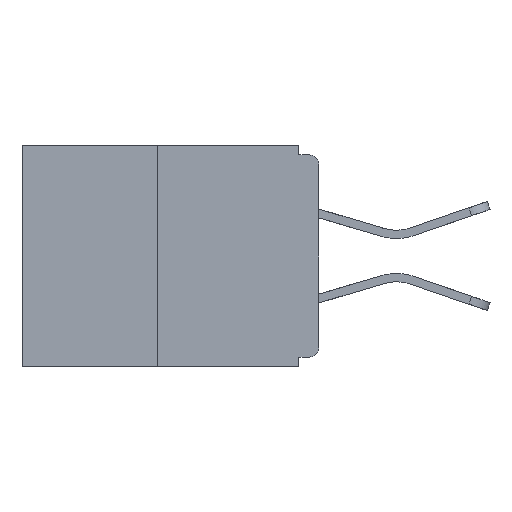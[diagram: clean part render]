
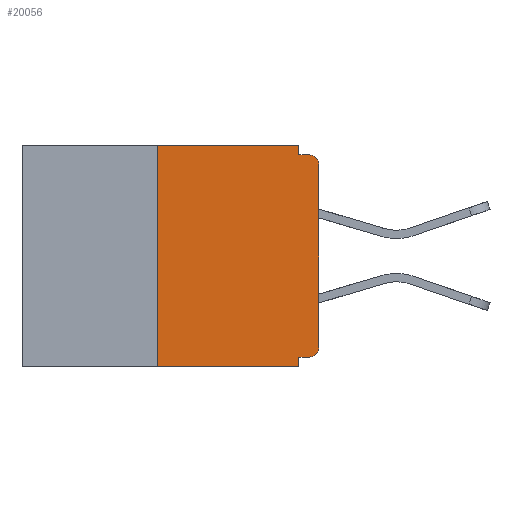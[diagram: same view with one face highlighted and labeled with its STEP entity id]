
A CAD part, left-side view. The second image highlights one B-rep face of the part: STEP entity #20056.
In plain terms, the highlighted planar face has unit normal (-1, 0, 0).
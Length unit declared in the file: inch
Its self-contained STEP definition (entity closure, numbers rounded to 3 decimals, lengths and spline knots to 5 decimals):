
#73 = EDGE_CURVE ( 'NONE', #3295, #20971, #19519, .T. ) ;
#151 = EDGE_CURVE ( 'NONE', #14253, #12249, #17177, .T. ) ;
#412 = LINE ( 'NONE', #5059, #3625 ) ;
#809 = VERTEX_POINT ( 'NONE', #22597 ) ;
#1054 = AXIS2_PLACEMENT_3D ( 'NONE', #11317, #15094, #13189 ) ;
#1122 = ORIENTED_EDGE ( 'NONE', *, *, #19939, .F. ) ;
#1125 = CARTESIAN_POINT ( 'NONE',  ( 0., 0.015, -0.313 ) ) ;
#1513 = EDGE_CURVE ( 'NONE', #12249, #12720, #15911, .T. ) ;
#1585 = VECTOR ( 'NONE', #18303, 39.37008 ) ;
#1712 = EDGE_CURVE ( 'NONE', #20971, #18091, #13228, .T. ) ;
#2370 = CARTESIAN_POINT ( 'NONE',  ( 0., 0.031, 0. ) ) ;
#2661 = CARTESIAN_POINT ( 'NONE',  ( 0., 0., -0.03 ) ) ;
#2832 = VERTEX_POINT ( 'NONE', #22808 ) ;
#2921 = AXIS2_PLACEMENT_3D ( 'NONE', #19587, #10387, #8738 ) ;
#3295 = VERTEX_POINT ( 'NONE', #2370 ) ;
#3625 = VECTOR ( 'NONE', #9280, 39.37008 ) ;
#3759 = DIRECTION ( 'NONE',  ( 0., -1., 0. ) ) ;
#4393 = CARTESIAN_POINT ( 'NONE',  ( 0., 0.031, -0.343 ) ) ;
#4500 = LINE ( 'NONE', #21960, #1585 ) ;
#4867 = DIRECTION ( 'NONE',  ( 0., 0., -1. ) ) ;
#5059 = CARTESIAN_POINT ( 'NONE',  ( 0., 0.031, -0.343 ) ) ;
#5072 = DIRECTION ( 'NONE',  ( 0., -1., 0. ) ) ;
#5205 = DIRECTION ( 'NONE',  ( -1., 0., 0. ) ) ;
#5251 = CARTESIAN_POINT ( 'NONE',  ( 0., 0.46, 0. ) ) ;
#6317 = VECTOR ( 'NONE', #10853, 39.37008 ) ;
#6762 = ORIENTED_EDGE ( 'NONE', *, *, #151, .T. ) ;
#6840 = DIRECTION ( 'NONE',  ( 0., 0., -1. ) ) ;
#6987 = EDGE_LOOP ( 'NONE', ( #1122, #18144, #11225, #13713, #10359, #6762, #20629, #10841, #23948, #20035 ) ) ;
#7115 = DIRECTION ( 'NONE',  ( 0., 0., 1. ) ) ;
#7247 = VECTOR ( 'NONE', #19652, 39.37008 ) ;
#7789 = VECTOR ( 'NONE', #4867, 39.37008 ) ;
#8685 = AXIS2_PLACEMENT_3D ( 'NONE', #1125, #5205, #6840 ) ;
#8738 = DIRECTION ( 'NONE',  ( 0., 0., -1. ) ) ;
#8984 = CARTESIAN_POINT ( 'NONE',  ( 0., 0., 0. ) ) ;
#9280 = DIRECTION ( 'NONE',  ( 0., 0., -1. ) ) ;
#9584 = EDGE_CURVE ( 'NONE', #16856, #2832, #4500, .T. ) ;
#10359 = ORIENTED_EDGE ( 'NONE', *, *, #20008, .F. ) ;
#10387 = DIRECTION ( 'NONE',  ( -1., 0., 0. ) ) ;
#10841 = ORIENTED_EDGE ( 'NONE', *, *, #15151, .T. ) ;
#10853 = DIRECTION ( 'NONE',  ( 0., 1., 0. ) ) ;
#11225 = ORIENTED_EDGE ( 'NONE', *, *, #19388, .T. ) ;
#11245 = VECTOR ( 'NONE', #5072, 39.37008 ) ;
#11317 = CARTESIAN_POINT ( 'NONE',  ( 0., 0.46, 0. ) ) ;
#12009 = CARTESIAN_POINT ( 'NONE',  ( 0., 0.015, -0.328 ) ) ;
#12249 = VERTEX_POINT ( 'NONE', #15370 ) ;
#12545 = CARTESIAN_POINT ( 'NONE',  ( 0., 0., -0.328 ) ) ;
#12720 = VERTEX_POINT ( 'NONE', #2661 ) ;
#12951 = PLANE ( 'NONE',  #1054 ) ;
#13189 = DIRECTION ( 'NONE',  ( 0., 0., -1. ) ) ;
#13228 = LINE ( 'NONE', #15161, #14723 ) ;
#13711 = CARTESIAN_POINT ( 'NONE',  ( 0., 0.031, -0.015 ) ) ;
#13713 = ORIENTED_EDGE ( 'NONE', *, *, #18027, .F. ) ;
#13948 = CARTESIAN_POINT ( 'NONE',  ( 0., 0.46, -0.343 ) ) ;
#14253 = VERTEX_POINT ( 'NONE', #12009 ) ;
#14723 = VECTOR ( 'NONE', #3759, 39.37008 ) ;
#15094 = DIRECTION ( 'NONE',  ( 1., 0., 0. ) ) ;
#15151 = EDGE_CURVE ( 'NONE', #12720, #18091, #20489, .T. ) ;
#15161 = CARTESIAN_POINT ( 'NONE',  ( 0., 0., -0.015 ) ) ;
#15163 = CARTESIAN_POINT ( 'NONE',  ( 0., 0.25, -0.343 ) ) ;
#15370 = CARTESIAN_POINT ( 'NONE',  ( 0., 0., -0.313 ) ) ;
#15911 = LINE ( 'NONE', #8984, #22402 ) ;
#16222 = CARTESIAN_POINT ( 'NONE',  ( 0., 0.031, 0. ) ) ;
#16253 = LINE ( 'NONE', #12545, #6317 ) ;
#16856 = VERTEX_POINT ( 'NONE', #15163 ) ;
#17177 = CIRCLE ( 'NONE', #8685, 0.015 ) ;
#18027 = EDGE_CURVE ( 'NONE', #809, #20224, #412, .T. ) ;
#18091 = VERTEX_POINT ( 'NONE', #22561 ) ;
#18144 = ORIENTED_EDGE ( 'NONE', *, *, #9584, .F. ) ;
#18303 = DIRECTION ( 'NONE',  ( 0., 0., 1. ) ) ;
#18648 = LINE ( 'NONE', #5251, #11245 ) ;
#19388 = EDGE_CURVE ( 'NONE', #16856, #20224, #20722, .T. ) ;
#19519 = LINE ( 'NONE', #16222, #7789 ) ;
#19587 = CARTESIAN_POINT ( 'NONE',  ( 0., 0.015, -0.03 ) ) ;
#19652 = DIRECTION ( 'NONE',  ( 0., -1., 0. ) ) ;
#19939 = EDGE_CURVE ( 'NONE', #2832, #3295, #18648, .T. ) ;
#20008 = EDGE_CURVE ( 'NONE', #14253, #809, #16253, .T. ) ;
#20035 = ORIENTED_EDGE ( 'NONE', *, *, #73, .F. ) ;
#20056 = ADVANCED_FACE ( 'NONE', ( #21834 ), #12951, .F. ) ;
#20224 = VERTEX_POINT ( 'NONE', #4393 ) ;
#20489 = CIRCLE ( 'NONE', #2921, 0.015 ) ;
#20629 = ORIENTED_EDGE ( 'NONE', *, *, #1513, .T. ) ;
#20722 = LINE ( 'NONE', #13948, #7247 ) ;
#20971 = VERTEX_POINT ( 'NONE', #13711 ) ;
#21834 = FACE_OUTER_BOUND ( 'NONE', #6987, .T. ) ;
#21960 = CARTESIAN_POINT ( 'NONE',  ( 0., 0.25, 0. ) ) ;
#22402 = VECTOR ( 'NONE', #7115, 39.37008 ) ;
#22561 = CARTESIAN_POINT ( 'NONE',  ( 0., 0.015, -0.015 ) ) ;
#22597 = CARTESIAN_POINT ( 'NONE',  ( 0., 0.031, -0.328 ) ) ;
#22808 = CARTESIAN_POINT ( 'NONE',  ( 0., 0.25, 0. ) ) ;
#23948 = ORIENTED_EDGE ( 'NONE', *, *, #1712, .F. ) ;
